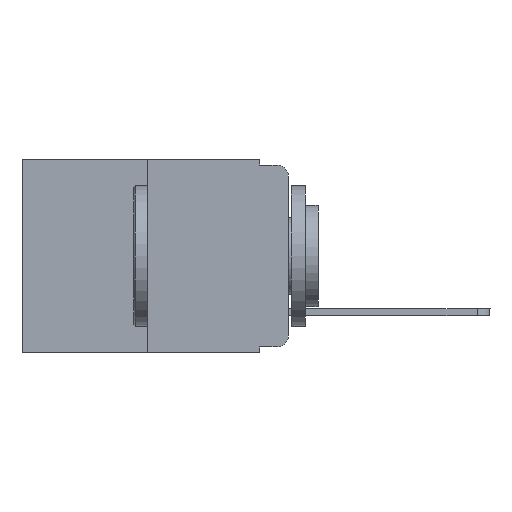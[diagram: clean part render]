
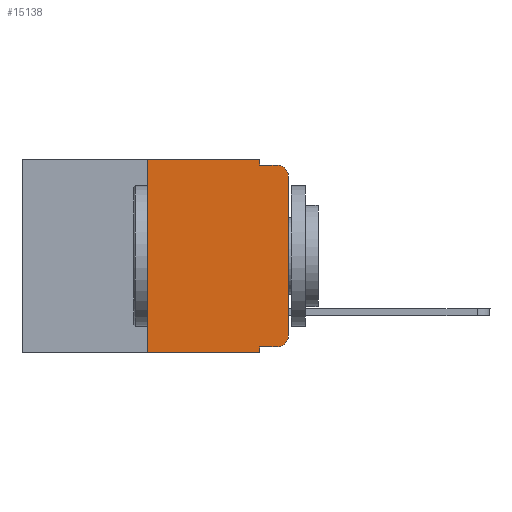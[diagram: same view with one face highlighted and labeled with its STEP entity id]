
A CAD part, left-side view. The second image highlights one B-rep face of the part: STEP entity #15138.
In plain terms, the highlighted planar face has unit normal (-1, 0, 0).
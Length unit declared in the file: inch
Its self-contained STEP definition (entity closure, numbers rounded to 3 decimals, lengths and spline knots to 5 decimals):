
#20 = CARTESIAN_POINT ( 'NONE',  ( 0., 0.051, 0. ) ) ;
#547 = LINE ( 'NONE', #15427, #14612 ) ;
#649 = VECTOR ( 'NONE', #12718, 39.37008 ) ;
#707 = DIRECTION ( 'NONE',  ( 1., 0., 0. ) ) ;
#1476 = CARTESIAN_POINT ( 'NONE',  ( 0., 0.051, -0.343 ) ) ;
#1518 = LINE ( 'NONE', #12865, #7638 ) ;
#2025 = ORIENTED_EDGE ( 'NONE', *, *, #4467, .F. ) ;
#2034 = CARTESIAN_POINT ( 'NONE',  ( 0., 0.473, -0.343 ) ) ;
#2275 = ORIENTED_EDGE ( 'NONE', *, *, #12796, .F. ) ;
#2472 = VECTOR ( 'NONE', #12542, 39.37008 ) ;
#2607 = EDGE_LOOP ( 'NONE', ( #2838, #2824, #10635, #2025, #2275, #3114, #9672, #13715, #5752, #9835 ) ) ;
#2824 = ORIENTED_EDGE ( 'NONE', *, *, #7005, .T. ) ;
#2838 = ORIENTED_EDGE ( 'NONE', *, *, #9680, .T. ) ;
#2858 = LINE ( 'NONE', #11269, #2472 ) ;
#3114 = ORIENTED_EDGE ( 'NONE', *, *, #14492, .F. ) ;
#3294 = CARTESIAN_POINT ( 'NONE',  ( 0., 0.473, 0. ) ) ;
#3405 = LINE ( 'NONE', #6752, #5118 ) ;
#3848 = VECTOR ( 'NONE', #9365, 39.37008 ) ;
#4168 = CARTESIAN_POINT ( 'NONE',  ( 0., 0.02, -0.01 ) ) ;
#4304 = CARTESIAN_POINT ( 'NONE',  ( 0., 0., -0.03 ) ) ;
#4383 = VERTEX_POINT ( 'NONE', #5830 ) ;
#4389 = CARTESIAN_POINT ( 'NONE',  ( 0., 0.051, -0.01 ) ) ;
#4467 = EDGE_CURVE ( 'NONE', #6551, #12230, #547, .T. ) ;
#4914 = CARTESIAN_POINT ( 'NONE',  ( 0., 0., 0. ) ) ;
#4949 = VECTOR ( 'NONE', #15428, 39.37008 ) ;
#5118 = VECTOR ( 'NONE', #10587, 39.37008 ) ;
#5225 = VERTEX_POINT ( 'NONE', #15533 ) ;
#5752 = ORIENTED_EDGE ( 'NONE', *, *, #13748, .T. ) ;
#5777 = EDGE_CURVE ( 'NONE', #5225, #11517, #6251, .T. ) ;
#5830 = CARTESIAN_POINT ( 'NONE',  ( 0., 0.051, -0.333 ) ) ;
#5964 = AXIS2_PLACEMENT_3D ( 'NONE', #7010, #10740, #8235 ) ;
#6233 = CARTESIAN_POINT ( 'NONE',  ( 0., 0.25, 0. ) ) ;
#6251 = CIRCLE ( 'NONE', #8516, 0.02 ) ;
#6478 = CIRCLE ( 'NONE', #5964, 0.02 ) ;
#6551 = VERTEX_POINT ( 'NONE', #20 ) ;
#6578 = AXIS2_PLACEMENT_3D ( 'NONE', #13965, #707, #13854 ) ;
#6752 = CARTESIAN_POINT ( 'NONE',  ( 0., 0.051, 0. ) ) ;
#6971 = LINE ( 'NONE', #4914, #649 ) ;
#7005 = EDGE_CURVE ( 'NONE', #14181, #13408, #6478, .T. ) ;
#7010 = CARTESIAN_POINT ( 'NONE',  ( 0., 0.02, -0.03 ) ) ;
#7474 = LINE ( 'NONE', #10774, #3848 ) ;
#7638 = VECTOR ( 'NONE', #14141, 39.37008 ) ;
#7783 = EDGE_CURVE ( 'NONE', #4383, #13940, #3405, .T. ) ;
#8147 = VERTEX_POINT ( 'NONE', #6233 ) ;
#8235 = DIRECTION ( 'NONE',  ( 0., 0., -1. ) ) ;
#8479 = VERTEX_POINT ( 'NONE', #14056 ) ;
#8516 = AXIS2_PLACEMENT_3D ( 'NONE', #14341, #9591, #9473 ) ;
#8782 = LINE ( 'NONE', #2034, #4949 ) ;
#9365 = DIRECTION ( 'NONE',  ( 0., -1., 0. ) ) ;
#9473 = DIRECTION ( 'NONE',  ( 0., 0., -1. ) ) ;
#9591 = DIRECTION ( 'NONE',  ( -1., 0., 0. ) ) ;
#9672 = ORIENTED_EDGE ( 'NONE', *, *, #15279, .T. ) ;
#9680 = EDGE_CURVE ( 'NONE', #11517, #14181, #6971, .T. ) ;
#9835 = ORIENTED_EDGE ( 'NONE', *, *, #5777, .T. ) ;
#10587 = DIRECTION ( 'NONE',  ( 0., 0., -1. ) ) ;
#10635 = ORIENTED_EDGE ( 'NONE', *, *, #14914, .F. ) ;
#10740 = DIRECTION ( 'NONE',  ( -1., 0., 0. ) ) ;
#10774 = CARTESIAN_POINT ( 'NONE',  ( 0., 0.051, -0.333 ) ) ;
#11023 = DIRECTION ( 'NONE',  ( 0., 0., -1. ) ) ;
#11269 = CARTESIAN_POINT ( 'NONE',  ( 0., 0.051, -0.01 ) ) ;
#11517 = VERTEX_POINT ( 'NONE', #11573 ) ;
#11573 = CARTESIAN_POINT ( 'NONE',  ( 0., 0., -0.313 ) ) ;
#11918 = DIRECTION ( 'NONE',  ( 0., -1., 0. ) ) ;
#12230 = VERTEX_POINT ( 'NONE', #4389 ) ;
#12542 = DIRECTION ( 'NONE',  ( 0., -1., 0. ) ) ;
#12718 = DIRECTION ( 'NONE',  ( 0., 0., 1. ) ) ;
#12747 = PLANE ( 'NONE',  #6578 ) ;
#12796 = EDGE_CURVE ( 'NONE', #8147, #6551, #15188, .T. ) ;
#12865 = CARTESIAN_POINT ( 'NONE',  ( 0., 0.25, 0. ) ) ;
#13408 = VERTEX_POINT ( 'NONE', #4168 ) ;
#13463 = FACE_OUTER_BOUND ( 'NONE', #2607, .T. ) ;
#13715 = ORIENTED_EDGE ( 'NONE', *, *, #7783, .F. ) ;
#13748 = EDGE_CURVE ( 'NONE', #4383, #5225, #7474, .T. ) ;
#13854 = DIRECTION ( 'NONE',  ( 0., 0., -1. ) ) ;
#13940 = VERTEX_POINT ( 'NONE', #1476 ) ;
#13965 = CARTESIAN_POINT ( 'NONE',  ( 0., 0.473, 0. ) ) ;
#14056 = CARTESIAN_POINT ( 'NONE',  ( 0., 0.25, -0.343 ) ) ;
#14141 = DIRECTION ( 'NONE',  ( 0., 0., 1. ) ) ;
#14181 = VERTEX_POINT ( 'NONE', #4304 ) ;
#14341 = CARTESIAN_POINT ( 'NONE',  ( 0., 0.02, -0.313 ) ) ;
#14426 = VECTOR ( 'NONE', #11918, 39.37008 ) ;
#14492 = EDGE_CURVE ( 'NONE', #8479, #8147, #1518, .T. ) ;
#14612 = VECTOR ( 'NONE', #11023, 39.37008 ) ;
#14914 = EDGE_CURVE ( 'NONE', #12230, #13408, #2858, .T. ) ;
#15138 = ADVANCED_FACE ( 'NONE', ( #13463 ), #12747, .F. ) ;
#15188 = LINE ( 'NONE', #3294, #14426 ) ;
#15279 = EDGE_CURVE ( 'NONE', #8479, #13940, #8782, .T. ) ;
#15427 = CARTESIAN_POINT ( 'NONE',  ( 0., 0.051, 0. ) ) ;
#15428 = DIRECTION ( 'NONE',  ( 0., -1., 0. ) ) ;
#15533 = CARTESIAN_POINT ( 'NONE',  ( 0., 0.02, -0.333 ) ) ;
